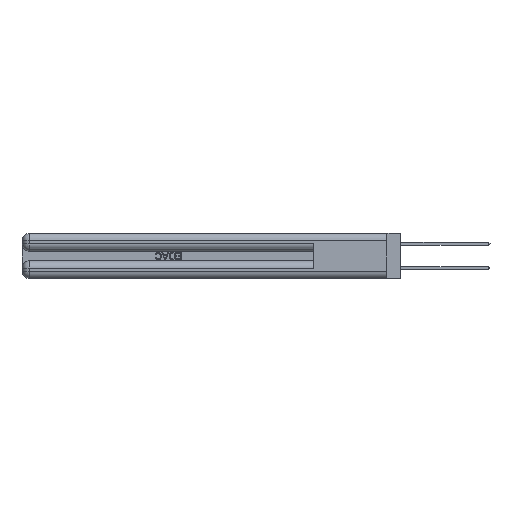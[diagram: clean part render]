
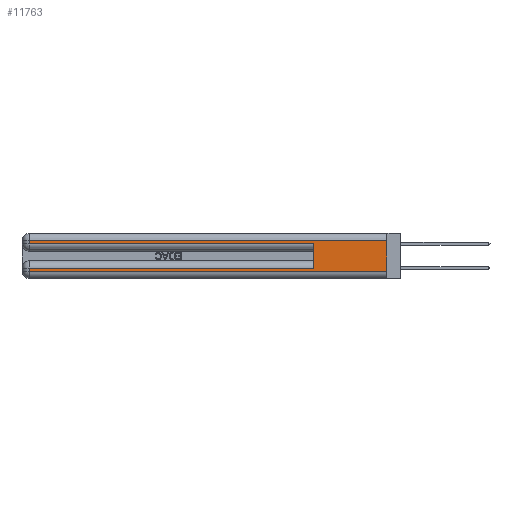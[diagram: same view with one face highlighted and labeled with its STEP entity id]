
A CAD part, left-side view. The second image highlights one B-rep face of the part: STEP entity #11763.
In plain terms, the highlighted planar face has unit normal (-1, 0, 0).
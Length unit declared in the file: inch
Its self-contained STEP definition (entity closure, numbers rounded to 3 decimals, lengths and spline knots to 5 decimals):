
#1411 = VERTEX_POINT ( 'NONE', #42967 ) ;
#1716 = VERTEX_POINT ( 'NONE', #19538 ) ;
#2323 = EDGE_CURVE ( 'NONE', #32314, #1411, #4213, .T. ) ;
#2500 = DIRECTION ( 'NONE',  ( 0., 0., 1. ) ) ;
#2955 = ORIENTED_EDGE ( 'NONE', *, *, #14182, .T. ) ;
#3281 = CARTESIAN_POINT ( 'NONE',  ( 0., 0., 0.31 ) ) ;
#3668 = VECTOR ( 'NONE', #6058, 39.37008 ) ;
#4213 = LINE ( 'NONE', #6138, #8346 ) ;
#4653 = PLANE ( 'NONE',  #8767 ) ;
#4822 = DIRECTION ( 'NONE',  ( 1., 0., 0. ) ) ;
#5744 = VECTOR ( 'NONE', #16208, 39.37008 ) ;
#6015 = EDGE_LOOP ( 'NONE', ( #35929, #44630, #36620, #2955, #39201, #47683, #38847, #27947 ) ) ;
#6058 = DIRECTION ( 'NONE',  ( 0., 0., -1. ) ) ;
#6138 = CARTESIAN_POINT ( 'NONE',  ( 0., 0.6, 0.145 ) ) ;
#7744 = VECTOR ( 'NONE', #9335, 39.37008 ) ;
#8100 = LINE ( 'NONE', #8454, #5744 ) ;
#8346 = VECTOR ( 'NONE', #2500, 39.37008 ) ;
#8454 = CARTESIAN_POINT ( 'NONE',  ( 0., 0., 0.085 ) ) ;
#8767 = AXIS2_PLACEMENT_3D ( 'NONE', #24152, #4822, #27805 ) ;
#9335 = DIRECTION ( 'NONE',  ( 0., -1., 0. ) ) ;
#9521 = DIRECTION ( 'NONE',  ( 0., 1., 0. ) ) ;
#10352 = CARTESIAN_POINT ( 'NONE',  ( 0., 2.94, 0.37 ) ) ;
#10815 = EDGE_CURVE ( 'NONE', #33546, #34205, #23193, .T. ) ;
#11763 = ADVANCED_FACE ( 'NONE', ( #43961 ), #4653, .F. ) ;
#12952 = LINE ( 'NONE', #32729, #15326 ) ;
#14182 = EDGE_CURVE ( 'NONE', #26311, #1411, #17789, .T. ) ;
#15326 = VECTOR ( 'NONE', #21453, 39.37008 ) ;
#16024 = CARTESIAN_POINT ( 'NONE',  ( 0., 0., 0.37 ) ) ;
#16208 = DIRECTION ( 'NONE',  ( 0., 1., 0. ) ) ;
#16290 = CARTESIAN_POINT ( 'NONE',  ( 0., 2.94, 0.285 ) ) ;
#17229 = CARTESIAN_POINT ( 'NONE',  ( 0., 0., 0.285 ) ) ;
#17789 = LINE ( 'NONE', #17229, #7744 ) ;
#19538 = CARTESIAN_POINT ( 'NONE',  ( 0., 2.94, 0.31 ) ) ;
#21233 = CARTESIAN_POINT ( 'NONE',  ( 0., 0., 0.31 ) ) ;
#21453 = DIRECTION ( 'NONE',  ( 0., -1., 0. ) ) ;
#21811 = EDGE_CURVE ( 'NONE', #41410, #1716, #41897, .T. ) ;
#22035 = VECTOR ( 'NONE', #45313, 39.37008 ) ;
#23193 = LINE ( 'NONE', #10352, #3668 ) ;
#24152 = CARTESIAN_POINT ( 'NONE',  ( 0., 0., 0.37 ) ) ;
#24223 = CARTESIAN_POINT ( 'NONE',  ( 0., 0.6, 0.085 ) ) ;
#25404 = CARTESIAN_POINT ( 'NONE',  ( 0., 2.94, 0.085 ) ) ;
#25787 = VECTOR ( 'NONE', #9521, 39.37008 ) ;
#25830 = EDGE_CURVE ( 'NONE', #34205, #48563, #12952, .T. ) ;
#26311 = VERTEX_POINT ( 'NONE', #16290 ) ;
#27147 = LINE ( 'NONE', #16024, #46254 ) ;
#27785 = DIRECTION ( 'NONE',  ( 0., 0., -1. ) ) ;
#27805 = DIRECTION ( 'NONE',  ( 0., 0., -1. ) ) ;
#27947 = ORIENTED_EDGE ( 'NONE', *, *, #25830, .T. ) ;
#29773 = CARTESIAN_POINT ( 'NONE',  ( 0., 2.94, 0.37 ) ) ;
#32314 = VERTEX_POINT ( 'NONE', #24223 ) ;
#32729 = CARTESIAN_POINT ( 'NONE',  ( 0., 0., 0.06 ) ) ;
#33546 = VERTEX_POINT ( 'NONE', #25404 ) ;
#34205 = VERTEX_POINT ( 'NONE', #41507 ) ;
#35929 = ORIENTED_EDGE ( 'NONE', *, *, #48523, .F. ) ;
#36620 = ORIENTED_EDGE ( 'NONE', *, *, #42736, .T. ) ;
#38847 = ORIENTED_EDGE ( 'NONE', *, *, #10815, .T. ) ;
#39201 = ORIENTED_EDGE ( 'NONE', *, *, #2323, .F. ) ;
#39579 = EDGE_CURVE ( 'NONE', #32314, #33546, #8100, .T. ) ;
#41410 = VERTEX_POINT ( 'NONE', #3281 ) ;
#41507 = CARTESIAN_POINT ( 'NONE',  ( 0., 2.94, 0.06 ) ) ;
#41897 = LINE ( 'NONE', #21233, #25787 ) ;
#42736 = EDGE_CURVE ( 'NONE', #1716, #26311, #45246, .T. ) ;
#42788 = CARTESIAN_POINT ( 'NONE',  ( 0., 0., 0.06 ) ) ;
#42967 = CARTESIAN_POINT ( 'NONE',  ( 0., 0.6, 0.285 ) ) ;
#43961 = FACE_OUTER_BOUND ( 'NONE', #6015, .T. ) ;
#44630 = ORIENTED_EDGE ( 'NONE', *, *, #21811, .T. ) ;
#45246 = LINE ( 'NONE', #29773, #22035 ) ;
#45313 = DIRECTION ( 'NONE',  ( 0., 0., -1. ) ) ;
#46254 = VECTOR ( 'NONE', #27785, 39.37008 ) ;
#47683 = ORIENTED_EDGE ( 'NONE', *, *, #39579, .T. ) ;
#48523 = EDGE_CURVE ( 'NONE', #41410, #48563, #27147, .T. ) ;
#48563 = VERTEX_POINT ( 'NONE', #42788 ) ;
